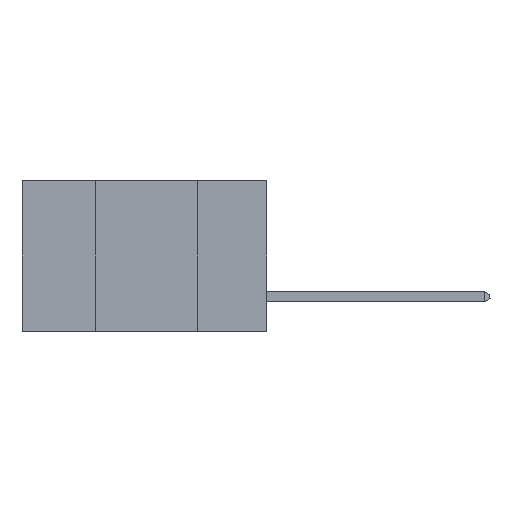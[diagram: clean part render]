
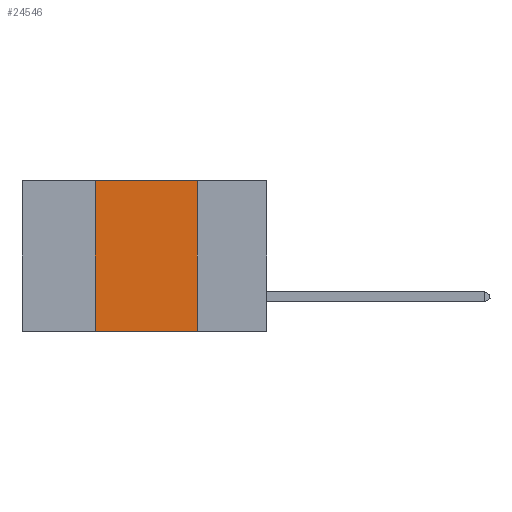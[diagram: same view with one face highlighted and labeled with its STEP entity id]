
A CAD part, left-side view. The second image highlights one B-rep face of the part: STEP entity #24546.
In plain terms, the highlighted planar face has unit normal (-1, 0, 0).
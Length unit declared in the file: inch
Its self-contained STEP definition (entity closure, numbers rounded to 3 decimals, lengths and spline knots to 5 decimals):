
#698 = ORIENTED_EDGE ( 'NONE', *, *, #24539, .T. ) ;
#1881 = EDGE_CURVE ( 'NONE', #6911, #8645, #12336, .T. ) ;
#1956 = PLANE ( 'NONE',  #25299 ) ;
#3083 = LINE ( 'NONE', #20173, #4864 ) ;
#4319 = CARTESIAN_POINT ( 'NONE',  ( 0., 0.17, 0. ) ) ;
#4522 = VERTEX_POINT ( 'NONE', #17179 ) ;
#4864 = VECTOR ( 'NONE', #11147, 39.37008 ) ;
#4991 = VERTEX_POINT ( 'NONE', #25777 ) ;
#6079 = EDGE_CURVE ( 'NONE', #4522, #6911, #13166, .T. ) ;
#6323 = CARTESIAN_POINT ( 'NONE',  ( 0., 0.6, 0. ) ) ;
#6911 = VERTEX_POINT ( 'NONE', #17295 ) ;
#8374 = DIRECTION ( 'NONE',  ( 0., 0., 1. ) ) ;
#8645 = VERTEX_POINT ( 'NONE', #4319 ) ;
#8905 = DIRECTION ( 'NONE',  ( 1., 0., 0. ) ) ;
#9241 = CARTESIAN_POINT ( 'NONE',  ( 0., 0.17, 0. ) ) ;
#11147 = DIRECTION ( 'NONE',  ( 0., -1., 0. ) ) ;
#12336 = LINE ( 'NONE', #6323, #17802 ) ;
#13166 = LINE ( 'NONE', #13268, #20422 ) ;
#13268 = CARTESIAN_POINT ( 'NONE',  ( 0., 0.42, 0. ) ) ;
#17179 = CARTESIAN_POINT ( 'NONE',  ( 0., 0.42, -0.37 ) ) ;
#17295 = CARTESIAN_POINT ( 'NONE',  ( 0., 0.42, 0. ) ) ;
#17656 = VECTOR ( 'NONE', #20717, 39.37008 ) ;
#17802 = VECTOR ( 'NONE', #18023, 39.37008 ) ;
#17980 = CARTESIAN_POINT ( 'NONE',  ( 0., 0.6, 0. ) ) ;
#18023 = DIRECTION ( 'NONE',  ( 0., -1., 0. ) ) ;
#19223 = ORIENTED_EDGE ( 'NONE', *, *, #6079, .F. ) ;
#20173 = CARTESIAN_POINT ( 'NONE',  ( 0., 0.6, -0.37 ) ) ;
#20422 = VECTOR ( 'NONE', #8374, 39.37008 ) ;
#20717 = DIRECTION ( 'NONE',  ( 0., 0., -1. ) ) ;
#20896 = LINE ( 'NONE', #9241, #17656 ) ;
#20910 = EDGE_LOOP ( 'NONE', ( #26208, #25030, #19223, #698 ) ) ;
#24033 = EDGE_CURVE ( 'NONE', #8645, #4991, #20896, .T. ) ;
#24539 = EDGE_CURVE ( 'NONE', #4522, #4991, #3083, .T. ) ;
#24546 = ADVANCED_FACE ( 'NONE', ( #26947 ), #1956, .F. ) ;
#24695 = DIRECTION ( 'NONE',  ( 0., 0., -1. ) ) ;
#25030 = ORIENTED_EDGE ( 'NONE', *, *, #1881, .F. ) ;
#25299 = AXIS2_PLACEMENT_3D ( 'NONE', #17980, #8905, #24695 ) ;
#25777 = CARTESIAN_POINT ( 'NONE',  ( 0., 0.17, -0.37 ) ) ;
#26208 = ORIENTED_EDGE ( 'NONE', *, *, #24033, .F. ) ;
#26947 = FACE_OUTER_BOUND ( 'NONE', #20910, .T. ) ;
